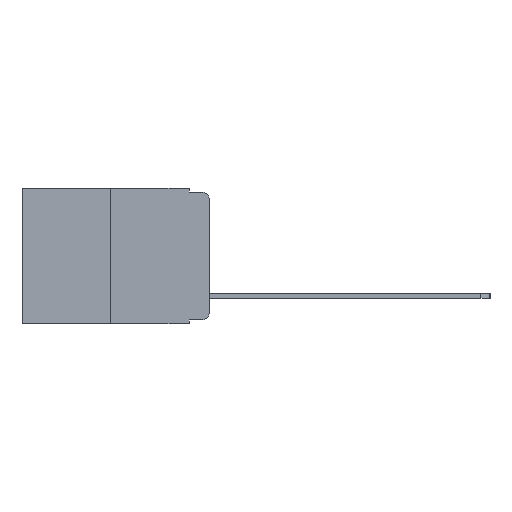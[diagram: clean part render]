
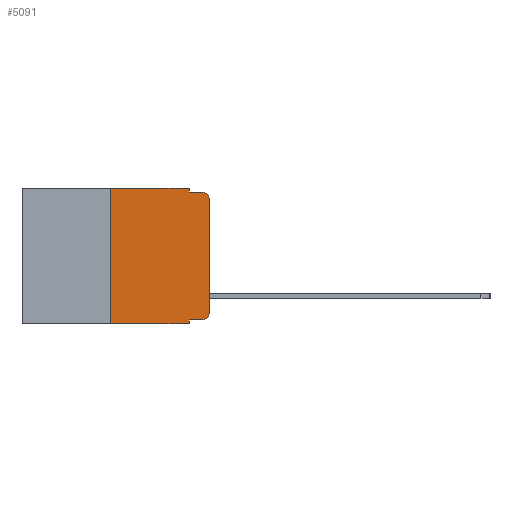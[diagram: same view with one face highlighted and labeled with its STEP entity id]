
A CAD part, left-side view. The second image highlights one B-rep face of the part: STEP entity #5091.
In plain terms, the highlighted planar face has unit normal (-1, 0, 0).
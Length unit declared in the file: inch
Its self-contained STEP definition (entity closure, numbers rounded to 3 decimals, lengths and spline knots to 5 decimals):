
#77 = DIRECTION ( 'NONE',  ( 0., 0., 1. ) ) ;
#501 = EDGE_CURVE ( 'NONE', #14154, #5172, #2302, .T. ) ;
#664 = DIRECTION ( 'NONE',  ( 0., 0., -1. ) ) ;
#772 = DIRECTION ( 'NONE',  ( -1., 0., 0. ) ) ;
#1358 = LINE ( 'NONE', #1696, #5577 ) ;
#1430 = LINE ( 'NONE', #6628, #16192 ) ;
#1581 = VECTOR ( 'NONE', #12914, 39.37008 ) ;
#1696 = CARTESIAN_POINT ( 'NONE',  ( 0., 0.25, 0. ) ) ;
#1755 = CARTESIAN_POINT ( 'NONE',  ( 0., 0.051, 0. ) ) ;
#1814 = DIRECTION ( 'NONE',  ( 0., -1., 0. ) ) ;
#2037 = LINE ( 'NONE', #3195, #10421 ) ;
#2087 = CARTESIAN_POINT ( 'NONE',  ( 0., 0.051, -0.333 ) ) ;
#2109 = VERTEX_POINT ( 'NONE', #12433 ) ;
#2302 = CIRCLE ( 'NONE', #8904, 0.02 ) ;
#2962 = EDGE_CURVE ( 'NONE', #5505, #10067, #16235, .T. ) ;
#3195 = CARTESIAN_POINT ( 'NONE',  ( 0., 0., 0. ) ) ;
#3205 = EDGE_LOOP ( 'NONE', ( #7040, #8018, #9703, #10710, #13153, #18343, #12905, #13936, #20056, #16899 ) ) ;
#3385 = EDGE_CURVE ( 'NONE', #5448, #4391, #4157, .T. ) ;
#3502 = CARTESIAN_POINT ( 'NONE',  ( 0., 0.051, 0. ) ) ;
#4157 = LINE ( 'NONE', #1755, #10895 ) ;
#4391 = VERTEX_POINT ( 'NONE', #4963 ) ;
#4440 = CARTESIAN_POINT ( 'NONE',  ( 0., 0.02, -0.03 ) ) ;
#4963 = CARTESIAN_POINT ( 'NONE',  ( 0., 0.051, -0.01 ) ) ;
#5091 = ADVANCED_FACE ( 'NONE', ( #9859 ), #13567, .F. ) ;
#5172 = VERTEX_POINT ( 'NONE', #13059 ) ;
#5448 = VERTEX_POINT ( 'NONE', #11580 ) ;
#5505 = VERTEX_POINT ( 'NONE', #13367 ) ;
#5577 = VECTOR ( 'NONE', #77, 39.37008 ) ;
#5594 = DIRECTION ( 'NONE',  ( 0., -1., 0. ) ) ;
#6628 = CARTESIAN_POINT ( 'NONE',  ( 0., 0.473, 0. ) ) ;
#6830 = EDGE_CURVE ( 'NONE', #10305, #5448, #1430, .T. ) ;
#6971 = CARTESIAN_POINT ( 'NONE',  ( 0., 0., -0.313 ) ) ;
#7040 = ORIENTED_EDGE ( 'NONE', *, *, #15087, .T. ) ;
#7275 = LINE ( 'NONE', #12807, #8255 ) ;
#7519 = LINE ( 'NONE', #12283, #19563 ) ;
#7578 = CARTESIAN_POINT ( 'NONE',  ( 0., 0.25, 0. ) ) ;
#7797 = DIRECTION ( 'NONE',  ( 0., -1., 0. ) ) ;
#7898 = EDGE_CURVE ( 'NONE', #12129, #2109, #7519, .T. ) ;
#8018 = ORIENTED_EDGE ( 'NONE', *, *, #501, .T. ) ;
#8137 = EDGE_CURVE ( 'NONE', #20258, #5505, #7275, .T. ) ;
#8255 = VECTOR ( 'NONE', #1814, 39.37008 ) ;
#8904 = AXIS2_PLACEMENT_3D ( 'NONE', #4440, #772, #664 ) ;
#9320 = EDGE_CURVE ( 'NONE', #20258, #2109, #17826, .T. ) ;
#9519 = VECTOR ( 'NONE', #5594, 39.37008 ) ;
#9703 = ORIENTED_EDGE ( 'NONE', *, *, #16981, .F. ) ;
#9859 = FACE_OUTER_BOUND ( 'NONE', #3205, .T. ) ;
#10067 = VERTEX_POINT ( 'NONE', #6971 ) ;
#10305 = VERTEX_POINT ( 'NONE', #7578 ) ;
#10421 = VECTOR ( 'NONE', #18919, 39.37008 ) ;
#10710 = ORIENTED_EDGE ( 'NONE', *, *, #3385, .F. ) ;
#10895 = VECTOR ( 'NONE', #14658, 39.37008 ) ;
#11580 = CARTESIAN_POINT ( 'NONE',  ( 0., 0.051, 0. ) ) ;
#12129 = VERTEX_POINT ( 'NONE', #12251 ) ;
#12251 = CARTESIAN_POINT ( 'NONE',  ( 0., 0.25, -0.343 ) ) ;
#12283 = CARTESIAN_POINT ( 'NONE',  ( 0., 0.473, -0.343 ) ) ;
#12433 = CARTESIAN_POINT ( 'NONE',  ( 0., 0.051, -0.343 ) ) ;
#12763 = AXIS2_PLACEMENT_3D ( 'NONE', #15420, #13634, #13630 ) ;
#12807 = CARTESIAN_POINT ( 'NONE',  ( 0., 0.051, -0.333 ) ) ;
#12905 = ORIENTED_EDGE ( 'NONE', *, *, #7898, .T. ) ;
#12914 = DIRECTION ( 'NONE',  ( 0., 0., -1. ) ) ;
#13059 = CARTESIAN_POINT ( 'NONE',  ( 0., 0.02, -0.01 ) ) ;
#13153 = ORIENTED_EDGE ( 'NONE', *, *, #6830, .F. ) ;
#13307 = CARTESIAN_POINT ( 'NONE',  ( 0., 0., -0.03 ) ) ;
#13367 = CARTESIAN_POINT ( 'NONE',  ( 0., 0.02, -0.333 ) ) ;
#13385 = CARTESIAN_POINT ( 'NONE',  ( 0., 0.051, -0.01 ) ) ;
#13567 = PLANE ( 'NONE',  #12763 ) ;
#13630 = DIRECTION ( 'NONE',  ( 0., 0., -1. ) ) ;
#13634 = DIRECTION ( 'NONE',  ( 1., 0., 0. ) ) ;
#13729 = LINE ( 'NONE', #13385, #9519 ) ;
#13890 = DIRECTION ( 'NONE',  ( 0., -1., 0. ) ) ;
#13936 = ORIENTED_EDGE ( 'NONE', *, *, #9320, .F. ) ;
#13949 = EDGE_CURVE ( 'NONE', #12129, #10305, #1358, .T. ) ;
#14154 = VERTEX_POINT ( 'NONE', #13307 ) ;
#14572 = DIRECTION ( 'NONE',  ( 0., 0., -1. ) ) ;
#14658 = DIRECTION ( 'NONE',  ( 0., 0., -1. ) ) ;
#15087 = EDGE_CURVE ( 'NONE', #10067, #14154, #2037, .T. ) ;
#15420 = CARTESIAN_POINT ( 'NONE',  ( 0., 0.473, 0. ) ) ;
#16192 = VECTOR ( 'NONE', #7797, 39.37008 ) ;
#16235 = CIRCLE ( 'NONE', #19444, 0.02 ) ;
#16279 = DIRECTION ( 'NONE',  ( -1., 0., 0. ) ) ;
#16287 = CARTESIAN_POINT ( 'NONE',  ( 0., 0.02, -0.313 ) ) ;
#16899 = ORIENTED_EDGE ( 'NONE', *, *, #2962, .T. ) ;
#16981 = EDGE_CURVE ( 'NONE', #4391, #5172, #13729, .T. ) ;
#17826 = LINE ( 'NONE', #3502, #1581 ) ;
#18343 = ORIENTED_EDGE ( 'NONE', *, *, #13949, .F. ) ;
#18919 = DIRECTION ( 'NONE',  ( 0., 0., 1. ) ) ;
#19444 = AXIS2_PLACEMENT_3D ( 'NONE', #16287, #16279, #14572 ) ;
#19563 = VECTOR ( 'NONE', #13890, 39.37008 ) ;
#20056 = ORIENTED_EDGE ( 'NONE', *, *, #8137, .T. ) ;
#20258 = VERTEX_POINT ( 'NONE', #2087 ) ;
